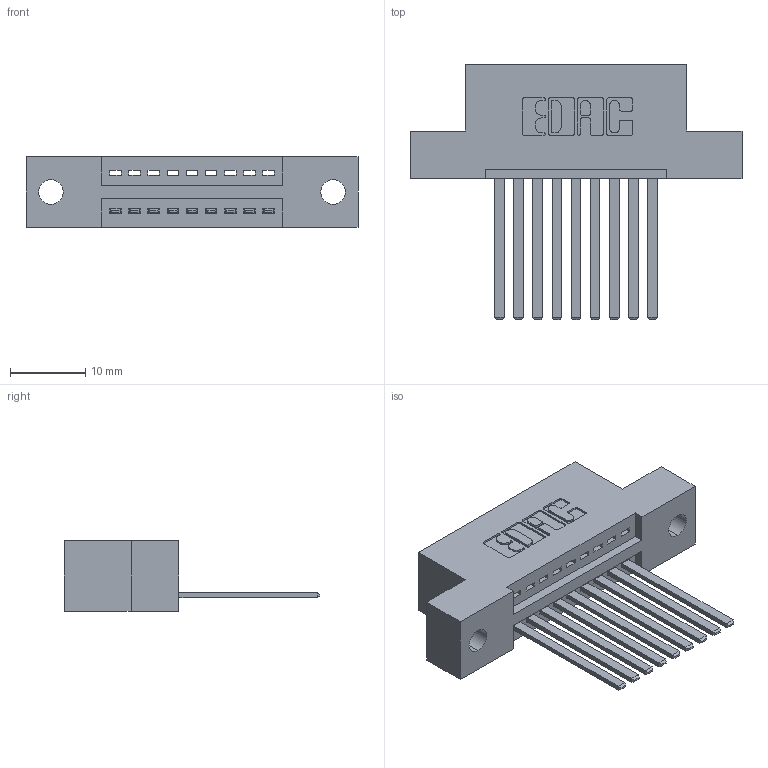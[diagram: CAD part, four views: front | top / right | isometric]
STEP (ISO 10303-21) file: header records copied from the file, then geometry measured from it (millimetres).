
FILE_DESCRIPTION (( 'STEP AP203' ), '1' );
FILE_NAME ('395-009-544-102.STEP', '2018-10-24T02:08:32', ( '' ), ( '' ), 'SwSTEP 2.0', 'SolidWorks 2016', '' );
FILE_SCHEMA (( 'CONFIG_CONTROL_DESIGN' ));
Length unit declared in the file: inch
Products named in the file (3): 345-292-001_345-293-144; 395-009-544-102; 345 Part_Flush Mounting Lugs - 0.128 Dia
Assembly tree (10 placements, depth 2):
  395-009-544-102
    345 Part_Flush Mounting Lugs - 0.128 Dia
    345-292-001_345-293-144  x9
Bounding box: 44.07 x 33.96 x 9.4 mm (x, y, z)
Volume: 3982.9 mm3; surface area: 4885.9 mm2
Topology: 10 solids, 10 shells, 594 faces, 1763 edges, 1162 vertices
Faces by surface type: plane 404, cylinder 190
Entity records: 11035 total; most frequent: CARTESIAN_POINT 1919, ORIENTED_EDGE 1862, DIRECTION 1721, EDGE_CURVE 931, LINE 767, VECTOR 767, VERTEX_POINT 618, AXIS2_PLACEMENT_3D 477
